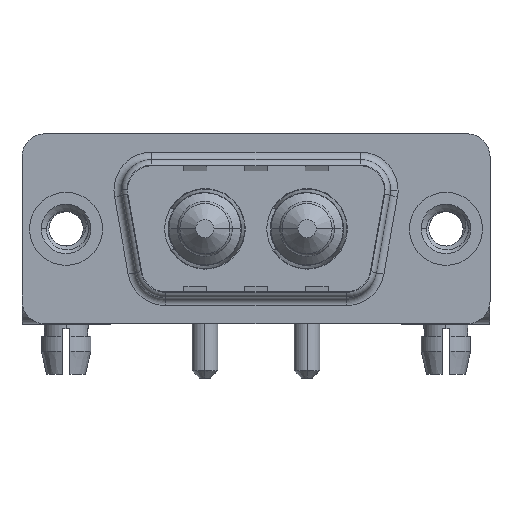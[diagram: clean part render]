
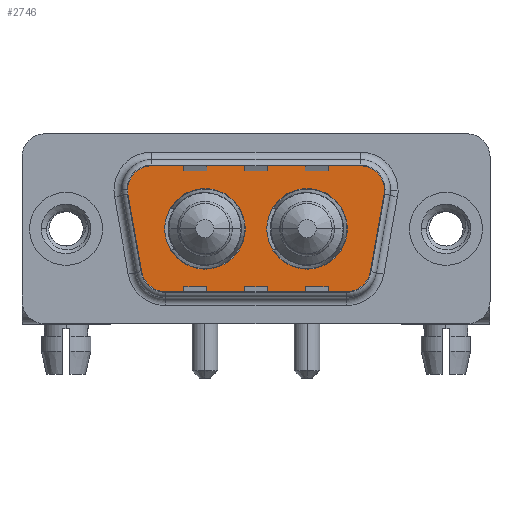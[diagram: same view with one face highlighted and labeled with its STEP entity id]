
A CAD part, top view. The second image highlights one B-rep face of the part: STEP entity #2746.
In plain terms, the highlighted planar face has unit normal (0, 0, 1).
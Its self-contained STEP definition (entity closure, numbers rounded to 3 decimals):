
#172 = EDGE_CURVE ( 'NONE', #8023, #9825, #764, .T. ) ;
#433 = EDGE_LOOP ( 'NONE', ( #10038, #12841, #6584, #7381, #1856, #5922, #4467, #11703, #6131 ) ) ;
#518 = EDGE_CURVE ( 'NONE', #4253, #6403, #12140, .T. ) ;
#764 = CIRCLE ( 'NONE', #2568, 2. ) ;
#969 = ORIENTED_EDGE ( 'NONE', *, *, #5181, .F. ) ;
#1021 = EDGE_CURVE ( 'NONE', #5099, #8023, #13632, .T. ) ;
#1151 = EDGE_CURVE ( 'NONE', #10395, #2784, #13406, .T. ) ;
#1340 = EDGE_CURVE ( 'NONE', #3390, #5099, #7942, .T. ) ;
#1455 = VECTOR ( 'NONE', #7356, 1000. ) ;
#1473 = DIRECTION ( 'NONE',  ( 0., 0., 1. ) ) ;
#1723 = EDGE_CURVE ( 'NONE', #12114, #10004, #5007, .T. ) ;
#1856 = ORIENTED_EDGE ( 'NONE', *, *, #3703, .T. ) ;
#2215 = EDGE_CURVE ( 'NONE', #4782, #5736, #9749, .T. ) ;
#2493 = DIRECTION ( 'NONE',  ( 1., 0., 0. ) ) ;
#2568 = AXIS2_PLACEMENT_3D ( 'NONE', #7881, #13402, #8094 ) ;
#2586 = CARTESIAN_POINT ( 'NONE',  ( 19.564, 4.9, 0. ) ) ;
#2646 = EDGE_CURVE ( 'NONE', #10004, #4253, #8984, .T. ) ;
#2746 = ADVANCED_FACE ( 'NONE', ( #6375, #4303, #8658 ), #13032, .T. ) ;
#2784 = VERTEX_POINT ( 'NONE', #6593 ) ;
#2976 = EDGE_LOOP ( 'NONE', ( #10703, #13695 ) ) ;
#3149 = CIRCLE ( 'NONE', #5421, 2.65 ) ;
#3310 = DIRECTION ( 'NONE',  ( 1., 0., 0. ) ) ;
#3345 = VECTOR ( 'NONE', #13993, 1000. ) ;
#3361 = CARTESIAN_POINT ( 'NONE',  ( 20.511, -3.247, 0. ) ) ;
#3390 = VERTEX_POINT ( 'NONE', #3361 ) ;
#3658 = DIRECTION ( 'NONE',  ( 0.174, 0.985, 0. ) ) ;
#3703 = EDGE_CURVE ( 'NONE', #9825, #12114, #6269, .T. ) ;
#3878 = CARTESIAN_POINT ( 'NONE',  ( 11.79, 0., 0. ) ) ;
#4081 = LINE ( 'NONE', #10440, #1455 ) ;
#4148 = DIRECTION ( 'NONE',  ( 1., 0., 0. ) ) ;
#4253 = VERTEX_POINT ( 'NONE', #10153 ) ;
#4303 = FACE_BOUND ( 'NONE', #10545, .T. ) ;
#4334 = CARTESIAN_POINT ( 'NONE',  ( 5.436, 4.9, 0. ) ) ;
#4467 = ORIENTED_EDGE ( 'NONE', *, *, #2646, .T. ) ;
#4661 = EDGE_CURVE ( 'NONE', #2784, #10395, #9280, .T. ) ;
#4663 = CARTESIAN_POINT ( 'NONE',  ( 21.534, 2.553, 0. ) ) ;
#4706 = CARTESIAN_POINT ( 'NONE',  ( 15.86, 0., 0. ) ) ;
#4782 = VERTEX_POINT ( 'NONE', #12711 ) ;
#4973 = EDGE_CURVE ( 'NONE', #6008, #3390, #11800, .T. ) ;
#5007 = CIRCLE ( 'NONE', #13013, 2. ) ;
#5097 = CARTESIAN_POINT ( 'NONE',  ( 21.564, 2.9, 0. ) ) ;
#5099 = VERTEX_POINT ( 'NONE', #13417 ) ;
#5181 = EDGE_CURVE ( 'NONE', #5736, #4782, #3149, .T. ) ;
#5241 = CARTESIAN_POINT ( 'NONE',  ( 18.541, -4.9, 0. ) ) ;
#5296 = CARTESIAN_POINT ( 'NONE',  ( 6.459, -2.9, 0. ) ) ;
#5413 = AXIS2_PLACEMENT_3D ( 'NONE', #13871, #9567, #13938 ) ;
#5421 = AXIS2_PLACEMENT_3D ( 'NONE', #11049, #8975, #13350 ) ;
#5567 = DIRECTION ( 'NONE',  ( 0., 0., 1. ) ) ;
#5635 = AXIS2_PLACEMENT_3D ( 'NONE', #4706, #5567, #2493 ) ;
#5736 = VERTEX_POINT ( 'NONE', #3878 ) ;
#5922 = ORIENTED_EDGE ( 'NONE', *, *, #1723, .T. ) ;
#6008 = VERTEX_POINT ( 'NONE', #5241 ) ;
#6131 = ORIENTED_EDGE ( 'NONE', *, *, #9920, .T. ) ;
#6269 = LINE ( 'NONE', #4334, #3345 ) ;
#6375 = FACE_BOUND ( 'NONE', #2976, .T. ) ;
#6403 = VERTEX_POINT ( 'NONE', #6413 ) ;
#6413 = CARTESIAN_POINT ( 'NONE',  ( 6.459, -4.9, 0. ) ) ;
#6584 = ORIENTED_EDGE ( 'NONE', *, *, #1021, .T. ) ;
#6593 = CARTESIAN_POINT ( 'NONE',  ( 13.21, 0., 0. ) ) ;
#6838 = DIRECTION ( 'NONE',  ( 0.174, -0.985, 0. ) ) ;
#7072 = ORIENTED_EDGE ( 'NONE', *, *, #2215, .F. ) ;
#7233 = CARTESIAN_POINT ( 'NONE',  ( 5.436, 4.9, 0. ) ) ;
#7335 = CARTESIAN_POINT ( 'NONE',  ( 18.541, -2.9, 0. ) ) ;
#7342 = DIRECTION ( 'NONE',  ( 1., 0., 0. ) ) ;
#7356 = DIRECTION ( 'NONE',  ( 1., 0., 0. ) ) ;
#7381 = ORIENTED_EDGE ( 'NONE', *, *, #172, .T. ) ;
#7405 = VECTOR ( 'NONE', #6838, 1000. ) ;
#7424 = DIRECTION ( 'NONE',  ( 0., 0., 1. ) ) ;
#7441 = DIRECTION ( 'NONE',  ( -1., 0., 0. ) ) ;
#7881 = CARTESIAN_POINT ( 'NONE',  ( 19.564, 2.9, 0. ) ) ;
#7942 = LINE ( 'NONE', #4663, #10936 ) ;
#8023 = VERTEX_POINT ( 'NONE', #5097 ) ;
#8039 = CARTESIAN_POINT ( 'NONE',  ( 3.466, 2.553, 0. ) ) ;
#8094 = DIRECTION ( 'NONE',  ( -1., 0., 0. ) ) ;
#8378 = AXIS2_PLACEMENT_3D ( 'NONE', #7335, #8472, #13997 ) ;
#8472 = DIRECTION ( 'NONE',  ( 0., 0., 1. ) ) ;
#8658 = FACE_OUTER_BOUND ( 'NONE', #433, .T. ) ;
#8722 = CARTESIAN_POINT ( 'NONE',  ( 18.541, -2.9, 0. ) ) ;
#8908 = AXIS2_PLACEMENT_3D ( 'NONE', #8722, #13103, #3310 ) ;
#8975 = DIRECTION ( 'NONE',  ( 0., 0., 1. ) ) ;
#8984 = LINE ( 'NONE', #8039, #7405 ) ;
#9280 = CIRCLE ( 'NONE', #5635, 2.65 ) ;
#9325 = AXIS2_PLACEMENT_3D ( 'NONE', #10106, #1473, #13012 ) ;
#9567 = DIRECTION ( 'NONE',  ( 0., 0., 1. ) ) ;
#9718 = CARTESIAN_POINT ( 'NONE',  ( 3.466, 2.553, 0. ) ) ;
#9749 = CIRCLE ( 'NONE', #12724, 2.65 ) ;
#9825 = VERTEX_POINT ( 'NONE', #2586 ) ;
#9920 = EDGE_CURVE ( 'NONE', #6403, #6008, #4081, .T. ) ;
#10004 = VERTEX_POINT ( 'NONE', #9718 ) ;
#10038 = ORIENTED_EDGE ( 'NONE', *, *, #4973, .T. ) ;
#10106 = CARTESIAN_POINT ( 'NONE',  ( 15.86, 0., 0. ) ) ;
#10153 = CARTESIAN_POINT ( 'NONE',  ( 4.489, -3.247, 0. ) ) ;
#10395 = VERTEX_POINT ( 'NONE', #13580 ) ;
#10440 = CARTESIAN_POINT ( 'NONE',  ( 6.459, -4.9, 0. ) ) ;
#10545 = EDGE_LOOP ( 'NONE', ( #969, #7072 ) ) ;
#10589 = DIRECTION ( 'NONE',  ( 0., 0., 1. ) ) ;
#10703 = ORIENTED_EDGE ( 'NONE', *, *, #1151, .F. ) ;
#10717 = CARTESIAN_POINT ( 'NONE',  ( 9.14, 0., 0. ) ) ;
#10936 = VECTOR ( 'NONE', #3658, 1000. ) ;
#11049 = CARTESIAN_POINT ( 'NONE',  ( 9.14, 0., 0. ) ) ;
#11703 = ORIENTED_EDGE ( 'NONE', *, *, #518, .T. ) ;
#11800 = CIRCLE ( 'NONE', #8378, 2. ) ;
#12021 = CARTESIAN_POINT ( 'NONE',  ( 5.436, 2.9, 0. ) ) ;
#12114 = VERTEX_POINT ( 'NONE', #7233 ) ;
#12140 = CIRCLE ( 'NONE', #13985, 2. ) ;
#12711 = CARTESIAN_POINT ( 'NONE',  ( 6.49, 0., 0. ) ) ;
#12724 = AXIS2_PLACEMENT_3D ( 'NONE', #10717, #7424, #7342 ) ;
#12841 = ORIENTED_EDGE ( 'NONE', *, *, #1340, .T. ) ;
#13012 = DIRECTION ( 'NONE',  ( 1., 0., 0. ) ) ;
#13013 = AXIS2_PLACEMENT_3D ( 'NONE', #12021, #13953, #4148 ) ;
#13032 = PLANE ( 'NONE',  #8908 ) ;
#13103 = DIRECTION ( 'NONE',  ( 0., 0., 1. ) ) ;
#13350 = DIRECTION ( 'NONE',  ( 1., 0., 0. ) ) ;
#13402 = DIRECTION ( 'NONE',  ( 0., 0., 1. ) ) ;
#13406 = CIRCLE ( 'NONE', #9325, 2.65 ) ;
#13417 = CARTESIAN_POINT ( 'NONE',  ( 21.534, 2.553, 0. ) ) ;
#13580 = CARTESIAN_POINT ( 'NONE',  ( 18.51, 0., 0. ) ) ;
#13632 = CIRCLE ( 'NONE', #5413, 2. ) ;
#13695 = ORIENTED_EDGE ( 'NONE', *, *, #4661, .F. ) ;
#13871 = CARTESIAN_POINT ( 'NONE',  ( 19.564, 2.9, 0. ) ) ;
#13938 = DIRECTION ( 'NONE',  ( -1., 0., 0. ) ) ;
#13953 = DIRECTION ( 'NONE',  ( 0., 0., 1. ) ) ;
#13985 = AXIS2_PLACEMENT_3D ( 'NONE', #5296, #10589, #7441 ) ;
#13993 = DIRECTION ( 'NONE',  ( -1., 0., 0. ) ) ;
#13997 = DIRECTION ( 'NONE',  ( 1., 0., 0. ) ) ;
